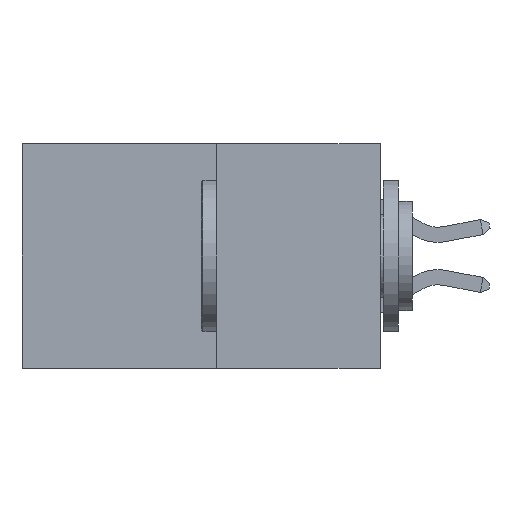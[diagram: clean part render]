
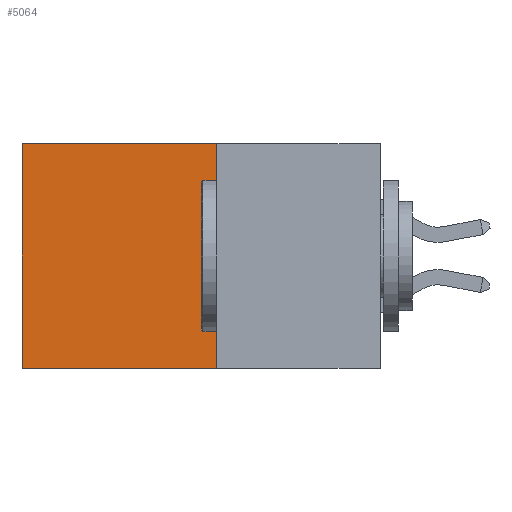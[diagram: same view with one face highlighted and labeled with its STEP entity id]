
A CAD part, left-side view. The second image highlights one B-rep face of the part: STEP entity #5064.
In plain terms, the highlighted planar face has unit normal (-1, 0, 0).
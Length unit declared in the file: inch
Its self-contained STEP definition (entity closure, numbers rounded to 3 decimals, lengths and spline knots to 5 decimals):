
#183 = AXIS2_PLACEMENT_3D ( 'NONE', #16981, #16804, #16724 ) ;
#203 = EDGE_CURVE ( 'NONE', #2196, #4441, #7403, .T. ) ;
#1210 = VECTOR ( 'NONE', #6935, 39.37008 ) ;
#1473 = ORIENTED_EDGE ( 'NONE', *, *, #15242, .F. ) ;
#1663 = LINE ( 'NONE', #6607, #1210 ) ;
#2196 = VERTEX_POINT ( 'NONE', #7608 ) ;
#2844 = CARTESIAN_POINT ( 'NONE',  ( 0.277, 0.27, -0.37 ) ) ;
#3667 = ORIENTED_EDGE ( 'NONE', *, *, #203, .F. ) ;
#4441 = VERTEX_POINT ( 'NONE', #4443 ) ;
#4443 = CARTESIAN_POINT ( 'NONE',  ( 0.277, 0.27, -0.37 ) ) ;
#5064 = ADVANCED_FACE ( 'NONE', ( #6355 ), #16837, .F. ) ;
#5152 = CARTESIAN_POINT ( 'NONE',  ( 0.277, 0.27, -0.37 ) ) ;
#6043 = LINE ( 'NONE', #2844, #13225 ) ;
#6147 = DIRECTION ( 'NONE',  ( 0., 0., -1. ) ) ;
#6192 = EDGE_LOOP ( 'NONE', ( #9370, #1473, #3667, #9304 ) ) ;
#6199 = CARTESIAN_POINT ( 'NONE',  ( 0.277, 0.59, -0.37 ) ) ;
#6355 = FACE_OUTER_BOUND ( 'NONE', #6192, .T. ) ;
#6607 = CARTESIAN_POINT ( 'NONE',  ( 0.277, 0.27, 0. ) ) ;
#6706 = EDGE_CURVE ( 'NONE', #2196, #16903, #1663, .T. ) ;
#6935 = DIRECTION ( 'NONE',  ( 0., 1., 0. ) ) ;
#7403 = LINE ( 'NONE', #5152, #11439 ) ;
#7608 = CARTESIAN_POINT ( 'NONE',  ( 0.277, 0.27, 0. ) ) ;
#7771 = EDGE_CURVE ( 'NONE', #16903, #10552, #7852, .T. ) ;
#7852 = LINE ( 'NONE', #6199, #8299 ) ;
#8299 = VECTOR ( 'NONE', #6147, 39.37008 ) ;
#9304 = ORIENTED_EDGE ( 'NONE', *, *, #6706, .T. ) ;
#9370 = ORIENTED_EDGE ( 'NONE', *, *, #7771, .T. ) ;
#10547 = CARTESIAN_POINT ( 'NONE',  ( 0.277, 0.59, 0. ) ) ;
#10552 = VERTEX_POINT ( 'NONE', #13988 ) ;
#11031 = DIRECTION ( 'NONE',  ( 0., 0., -1. ) ) ;
#11439 = VECTOR ( 'NONE', #11031, 39.37008 ) ;
#13225 = VECTOR ( 'NONE', #15021, 39.37008 ) ;
#13988 = CARTESIAN_POINT ( 'NONE',  ( 0.277, 0.59, -0.37 ) ) ;
#15021 = DIRECTION ( 'NONE',  ( 0., 1., 0. ) ) ;
#15242 = EDGE_CURVE ( 'NONE', #4441, #10552, #6043, .T. ) ;
#16724 = DIRECTION ( 'NONE',  ( 0., 0., -1. ) ) ;
#16804 = DIRECTION ( 'NONE',  ( 1., 0., 0. ) ) ;
#16837 = PLANE ( 'NONE',  #183 ) ;
#16903 = VERTEX_POINT ( 'NONE', #10547 ) ;
#16981 = CARTESIAN_POINT ( 'NONE',  ( 0.277, 0.27, -0.37 ) ) ;
